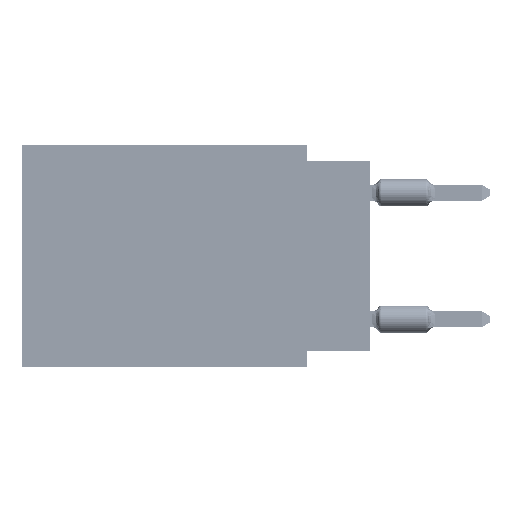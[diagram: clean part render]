
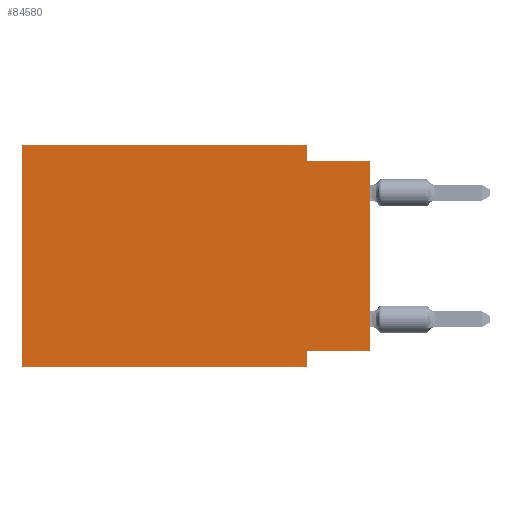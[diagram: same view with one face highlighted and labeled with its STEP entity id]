
A CAD part, left-side view. The second image highlights one B-rep face of the part: STEP entity #84580.
In plain terms, the highlighted planar face has unit normal (-1, 0, 0).
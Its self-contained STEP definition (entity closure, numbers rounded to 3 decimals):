
#110 = EDGE_CURVE ( 'NONE', #58346, #62849, #60686, .T. ) ;
#3391 = LINE ( 'NONE', #59925, #5810 ) ;
#5810 = VECTOR ( 'NONE', #99688, 1000. ) ;
#6855 = ORIENTED_EDGE ( 'NONE', *, *, #11029, .F. ) ;
#7508 = VERTEX_POINT ( 'NONE', #67005 ) ;
#7605 = CARTESIAN_POINT ( 'NONE',  ( 0., 2.54, 0. ) ) ;
#9076 = CARTESIAN_POINT ( 'NONE',  ( 0., 2.54, -8.89 ) ) ;
#10651 = VECTOR ( 'NONE', #71091, 1000. ) ;
#11029 = EDGE_CURVE ( 'NONE', #82640, #58217, #39179, .T. ) ;
#12772 = EDGE_CURVE ( 'NONE', #7508, #62849, #3391, .T. ) ;
#16043 = FACE_OUTER_BOUND ( 'NONE', #40701, .T. ) ;
#16241 = CARTESIAN_POINT ( 'NONE',  ( 0., 0., -0.635 ) ) ;
#18168 = EDGE_CURVE ( 'NONE', #44366, #7508, #56275, .T. ) ;
#18969 = ORIENTED_EDGE ( 'NONE', *, *, #12772, .F. ) ;
#20730 = VERTEX_POINT ( 'NONE', #46004 ) ;
#23240 = DIRECTION ( 'NONE',  ( 0., -1., 0. ) ) ;
#26680 = VECTOR ( 'NONE', #30927, 1000. ) ;
#26760 = EDGE_CURVE ( 'NONE', #98245, #44366, #75099, .T. ) ;
#27004 = ORIENTED_EDGE ( 'NONE', *, *, #91480, .T. ) ;
#29696 = DIRECTION ( 'NONE',  ( 0., 0., -1. ) ) ;
#30314 = CARTESIAN_POINT ( 'NONE',  ( 0., 0., 0. ) ) ;
#30927 = DIRECTION ( 'NONE',  ( 0., 0., 1. ) ) ;
#31785 = CARTESIAN_POINT ( 'NONE',  ( 0., 2.54, -8.255 ) ) ;
#31823 = ORIENTED_EDGE ( 'NONE', *, *, #26760, .F. ) ;
#32212 = VECTOR ( 'NONE', #99940, 1000. ) ;
#34974 = CARTESIAN_POINT ( 'NONE',  ( 0., 13.97, 0. ) ) ;
#36180 = CARTESIAN_POINT ( 'NONE',  ( 0., 13.97, 0. ) ) ;
#36262 = CARTESIAN_POINT ( 'NONE',  ( 0., 0., -8.255 ) ) ;
#37999 = DIRECTION ( 'NONE',  ( 0., 1., 0. ) ) ;
#39179 = LINE ( 'NONE', #63769, #10651 ) ;
#40701 = EDGE_LOOP ( 'NONE', ( #80490, #18969, #99238, #31823, #77545, #27004, #6855, #71612 ) ) ;
#44366 = VERTEX_POINT ( 'NONE', #76398 ) ;
#44503 = DIRECTION ( 'NONE',  ( 0., -1., 0. ) ) ;
#46004 = CARTESIAN_POINT ( 'NONE',  ( 0., 13.97, -8.89 ) ) ;
#47967 = PLANE ( 'NONE',  #71270 ) ;
#51831 = LINE ( 'NONE', #52336, #53558 ) ;
#52336 = CARTESIAN_POINT ( 'NONE',  ( 0., 13.97, -8.89 ) ) ;
#53558 = VECTOR ( 'NONE', #44503, 1000. ) ;
#54734 = DIRECTION ( 'NONE',  ( 0., 0., -1. ) ) ;
#54991 = VECTOR ( 'NONE', #54734, 1000. ) ;
#56275 = LINE ( 'NONE', #7605, #54991 ) ;
#58217 = VERTEX_POINT ( 'NONE', #9076 ) ;
#58346 = VERTEX_POINT ( 'NONE', #36262 ) ;
#59925 = CARTESIAN_POINT ( 'NONE',  ( 0., 0., -0.635 ) ) ;
#60013 = VECTOR ( 'NONE', #37999, 1000. ) ;
#60686 = LINE ( 'NONE', #30314, #32212 ) ;
#61495 = CARTESIAN_POINT ( 'NONE',  ( 0., 13.97, 0. ) ) ;
#62849 = VERTEX_POINT ( 'NONE', #16241 ) ;
#63099 = LINE ( 'NONE', #93459, #60013 ) ;
#63769 = CARTESIAN_POINT ( 'NONE',  ( 0., 2.54, -8.89 ) ) ;
#67005 = CARTESIAN_POINT ( 'NONE',  ( 0., 2.54, -0.635 ) ) ;
#71091 = DIRECTION ( 'NONE',  ( 0., 0., -1. ) ) ;
#71270 = AXIS2_PLACEMENT_3D ( 'NONE', #79874, #101386, #29696 ) ;
#71612 = ORIENTED_EDGE ( 'NONE', *, *, #93336, .F. ) ;
#75099 = LINE ( 'NONE', #61495, #75784 ) ;
#75784 = VECTOR ( 'NONE', #23240, 1000. ) ;
#75934 = LINE ( 'NONE', #36180, #26680 ) ;
#76398 = CARTESIAN_POINT ( 'NONE',  ( 0., 2.54, 0. ) ) ;
#77545 = ORIENTED_EDGE ( 'NONE', *, *, #94245, .F. ) ;
#79874 = CARTESIAN_POINT ( 'NONE',  ( 0., 13.97, 0. ) ) ;
#80490 = ORIENTED_EDGE ( 'NONE', *, *, #110, .T. ) ;
#82640 = VERTEX_POINT ( 'NONE', #31785 ) ;
#84580 = ADVANCED_FACE ( 'NONE', ( #16043 ), #47967, .F. ) ;
#91480 = EDGE_CURVE ( 'NONE', #20730, #58217, #51831, .T. ) ;
#93336 = EDGE_CURVE ( 'NONE', #58346, #82640, #63099, .T. ) ;
#93459 = CARTESIAN_POINT ( 'NONE',  ( 0., 0., -8.255 ) ) ;
#94245 = EDGE_CURVE ( 'NONE', #20730, #98245, #75934, .T. ) ;
#98245 = VERTEX_POINT ( 'NONE', #34974 ) ;
#99238 = ORIENTED_EDGE ( 'NONE', *, *, #18168, .F. ) ;
#99688 = DIRECTION ( 'NONE',  ( 0., -1., 0. ) ) ;
#99940 = DIRECTION ( 'NONE',  ( 0., 0., 1. ) ) ;
#101386 = DIRECTION ( 'NONE',  ( 1., 0., 0. ) ) ;
